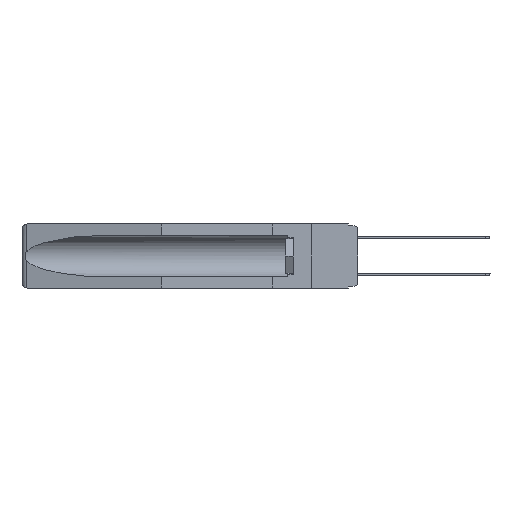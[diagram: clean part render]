
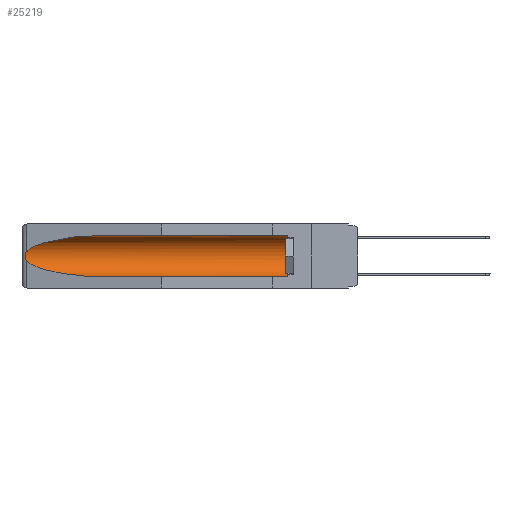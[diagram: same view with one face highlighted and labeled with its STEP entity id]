
A CAD part, left-side view. The second image highlights one B-rep face of the part: STEP entity #25219.
In plain terms, the highlighted cylindrical face has radius 2.857 mm (diameter 5.715 mm), a partial arc.
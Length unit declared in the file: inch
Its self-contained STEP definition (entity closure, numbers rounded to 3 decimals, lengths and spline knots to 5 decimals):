
#775 = CARTESIAN_POINT ( 'NONE',  ( 0.25451, 1.48313, -0.24835 ) ) ;
#946 = CARTESIAN_POINT ( 'NONE',  ( 0.26537, 1.52718, -0.14972 ) ) ;
#1285 = VERTEX_POINT ( 'NONE', #13801 ) ;
#2013 = AXIS2_PLACEMENT_3D ( 'NONE', #5428, #7799, #7925 ) ;
#2355 = ORIENTED_EDGE ( 'NONE', *, *, #7373, .T. ) ;
#2538 = DIRECTION ( 'NONE',  ( 0., 0., 1. ) ) ;
#3196 = ORIENTED_EDGE ( 'NONE', *, *, #4724, .F. ) ;
#3850 = CYLINDRICAL_SURFACE ( 'NONE', #2013, 0.1125 ) ;
#4724 = EDGE_CURVE ( 'NONE', #19970, #1285, #11018, .T. ) ;
#4908 = VERTEX_POINT ( 'NONE', #18737 ) ;
#4975 = DIRECTION ( 'NONE',  ( 0., 1., 0. ) ) ;
#5428 = CARTESIAN_POINT ( 'NONE',  ( 0.155, -0.30754, -0.1715 ) ) ;
#5806 = EDGE_CURVE ( 'NONE', #4908, #1285, #22168, .T. ) ;
#6902 = CARTESIAN_POINT ( 'NONE',  ( 0.155, 1.07973, -0.059 ) ) ;
#6995 = CARTESIAN_POINT ( 'NONE',  ( 0.26655, 1.53094, -0.18657 ) ) ;
#7074 = CARTESIAN_POINT ( 'NONE',  ( 0.155, -0.30754, -0.284 ) ) ;
#7284 = CIRCLE ( 'NONE', #19885, 0.1125 ) ;
#7373 = EDGE_CURVE ( 'NONE', #18076, #13678, #15086, .T. ) ;
#7504 = VECTOR ( 'NONE', #4975, 39.37008 ) ;
#7739 =( BOUNDED_CURVE ( )  B_SPLINE_CURVE ( 3, ( #17579, #11382, #9676, #23631 ),
 .UNSPECIFIED., .F., .T. ) 
 B_SPLINE_CURVE_WITH_KNOTS ( ( 4, 4 ),
 ( 4.71239, 6.08839 ),
 .UNSPECIFIED. ) 
 CURVE ( )  GEOMETRIC_REPRESENTATION_ITEM ( )  RATIONAL_B_SPLINE_CURVE ( ( 1., 0.848, 0.848, 1. ) ) 
 REPRESENTATION_ITEM ( '' )  );
#7799 = DIRECTION ( 'NONE',  ( 0., 1., 0. ) ) ;
#7857 = B_SPLINE_CURVE_WITH_KNOTS ( 'NONE', 3,
 ( #946, #14596, #8587, #14873, #16469, #12640, #8711, #6995, #14989, #22644 ),
 .UNSPECIFIED., .F., .F.,
 ( 4, 2, 2, 2, 4 ),
 ( 0., 0.00029, 0.00058, 0.00087, 0.00117 ),
 .UNSPECIFIED. ) ;
#7925 = DIRECTION ( 'NONE',  ( 0., 0., 1. ) ) ;
#7979 = ORIENTED_EDGE ( 'NONE', *, *, #21115, .T. ) ;
#8549 = CARTESIAN_POINT ( 'NONE',  ( 0.155, 1.07973, -0.284 ) ) ;
#8587 = CARTESIAN_POINT ( 'NONE',  ( 0.26654, 1.53092, -0.15636 ) ) ;
#8711 = CARTESIAN_POINT ( 'NONE',  ( 0.2673, 1.53269, -0.17917 ) ) ;
#9494 = ORIENTED_EDGE ( 'NONE', *, *, #23088, .T. ) ;
#9545 = CARTESIAN_POINT ( 'NONE',  ( 0.155, 0.126, -0.284 ) ) ;
#9676 = CARTESIAN_POINT ( 'NONE',  ( 0.25451, 1.48313, -0.09465 ) ) ;
#10258 = VERTEX_POINT ( 'NONE', #19050 ) ;
#11018 = LINE ( 'NONE', #7074, #7504 ) ;
#11382 = CARTESIAN_POINT ( 'NONE',  ( 0.21114, 1.30732, -0.059 ) ) ;
#12282 = ORIENTED_EDGE ( 'NONE', *, *, #14115, .T. ) ;
#12601 = CARTESIAN_POINT ( 'NONE',  ( 0.26537, 1.52718, -0.19328 ) ) ;
#12640 = CARTESIAN_POINT ( 'NONE',  ( 0.2675, 1.53308, -0.17534 ) ) ;
#12850 = CARTESIAN_POINT ( 'NONE',  ( 0.155, 0.126, -0.059 ) ) ;
#13678 = VERTEX_POINT ( 'NONE', #6902 ) ;
#13690 = FACE_OUTER_BOUND ( 'NONE', #14838, .T. ) ;
#13801 = CARTESIAN_POINT ( 'NONE',  ( 0.155, 1.07973, -0.284 ) ) ;
#14115 = EDGE_CURVE ( 'NONE', #10258, #4908, #7857, .T. ) ;
#14484 = CARTESIAN_POINT ( 'NONE',  ( 0.155, 0.126, -0.1715 ) ) ;
#14596 = CARTESIAN_POINT ( 'NONE',  ( 0.26597, 1.52961, -0.15275 ) ) ;
#14838 = EDGE_LOOP ( 'NONE', ( #7979, #12282, #23778, #3196, #9494, #2355 ) ) ;
#14873 = CARTESIAN_POINT ( 'NONE',  ( 0.2673, 1.5327, -0.16383 ) ) ;
#14989 = CARTESIAN_POINT ( 'NONE',  ( 0.26597, 1.5296, -0.19026 ) ) ;
#15086 = LINE ( 'NONE', #25512, #19869 ) ;
#15228 = DIRECTION ( 'NONE',  ( 0., 1., 0. ) ) ;
#16469 = CARTESIAN_POINT ( 'NONE',  ( 0.2675, 1.53308, -0.16763 ) ) ;
#17579 = CARTESIAN_POINT ( 'NONE',  ( 0.155, 1.07973, -0.059 ) ) ;
#18076 = VERTEX_POINT ( 'NONE', #12850 ) ;
#18544 = CARTESIAN_POINT ( 'NONE',  ( 0.21114, 1.30732, -0.284 ) ) ;
#18737 = CARTESIAN_POINT ( 'NONE',  ( 0.26537, 1.52718, -0.19328 ) ) ;
#19050 = CARTESIAN_POINT ( 'NONE',  ( 0.26537, 1.52718, -0.14972 ) ) ;
#19869 = VECTOR ( 'NONE', #15228, 39.37008 ) ;
#19885 = AXIS2_PLACEMENT_3D ( 'NONE', #14484, #23045, #2538 ) ;
#19970 = VERTEX_POINT ( 'NONE', #9545 ) ;
#21115 = EDGE_CURVE ( 'NONE', #13678, #10258, #7739, .T. ) ;
#22168 =( BOUNDED_CURVE ( )  B_SPLINE_CURVE ( 3, ( #12601, #775, #18544, #8549 ),
 .UNSPECIFIED., .F., .F. ) 
 B_SPLINE_CURVE_WITH_KNOTS ( ( 4, 4 ),
 ( 0.1948, 1.5708 ),
 .UNSPECIFIED. ) 
 CURVE ( )  GEOMETRIC_REPRESENTATION_ITEM ( )  RATIONAL_B_SPLINE_CURVE ( ( 1., 0.848, 0.848, 1. ) ) 
 REPRESENTATION_ITEM ( '' )  );
#22644 = CARTESIAN_POINT ( 'NONE',  ( 0.26537, 1.52718, -0.19328 ) ) ;
#23045 = DIRECTION ( 'NONE',  ( 0., -1., 0. ) ) ;
#23088 = EDGE_CURVE ( 'NONE', #19970, #18076, #7284, .T. ) ;
#23631 = CARTESIAN_POINT ( 'NONE',  ( 0.26537, 1.52718, -0.14972 ) ) ;
#23778 = ORIENTED_EDGE ( 'NONE', *, *, #5806, .T. ) ;
#25219 = ADVANCED_FACE ( 'NONE', ( #13690 ), #3850, .F. ) ;
#25512 = CARTESIAN_POINT ( 'NONE',  ( 0.155, -0.30754, -0.059 ) ) ;
